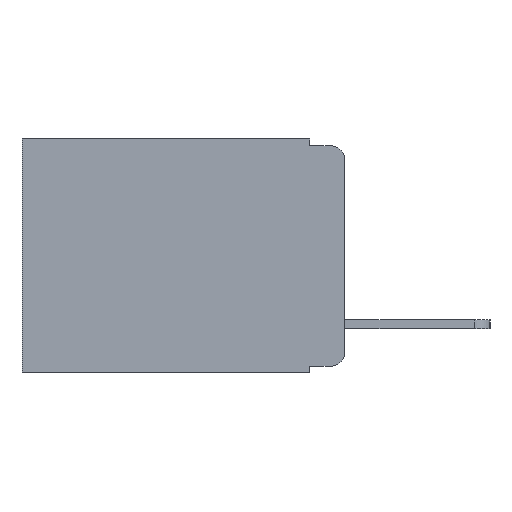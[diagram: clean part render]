
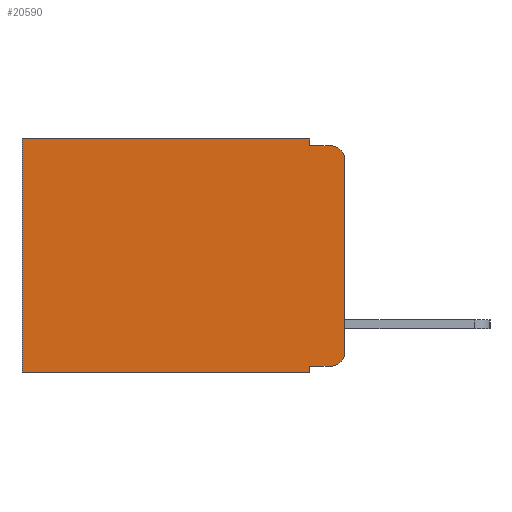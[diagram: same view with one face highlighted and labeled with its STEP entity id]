
A CAD part, left-side view. The second image highlights one B-rep face of the part: STEP entity #20590.
In plain terms, the highlighted planar face has unit normal (-1, 0, 0).
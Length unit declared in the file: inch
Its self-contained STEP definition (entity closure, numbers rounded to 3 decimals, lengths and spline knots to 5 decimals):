
#118 = CARTESIAN_POINT ( 'NONE',  ( 0.298, 0.051, -0.343 ) ) ;
#683 = CARTESIAN_POINT ( 'NONE',  ( 0.298, 0., 0. ) ) ;
#1264 = CARTESIAN_POINT ( 'NONE',  ( 0.298, 0.02, -0.03 ) ) ;
#1392 = VERTEX_POINT ( 'NONE', #2136 ) ;
#1413 = CARTESIAN_POINT ( 'NONE',  ( 0.298, 0.051, 0. ) ) ;
#1596 = CARTESIAN_POINT ( 'NONE',  ( 0.298, 0.051, -0.333 ) ) ;
#1978 = VERTEX_POINT ( 'NONE', #17481 ) ;
#2136 = CARTESIAN_POINT ( 'NONE',  ( 0.298, 0., -0.03 ) ) ;
#2285 = VERTEX_POINT ( 'NONE', #7405 ) ;
#2499 = VERTEX_POINT ( 'NONE', #1596 ) ;
#2525 = VERTEX_POINT ( 'NONE', #118 ) ;
#2598 = DIRECTION ( 'NONE',  ( 1., 0., 0. ) ) ;
#2883 = VERTEX_POINT ( 'NONE', #4368 ) ;
#3178 = DIRECTION ( 'NONE',  ( 0., 0., -1. ) ) ;
#3621 = EDGE_CURVE ( 'NONE', #1392, #4346, #22927, .T. ) ;
#4268 = EDGE_CURVE ( 'NONE', #1978, #2285, #23722, .T. ) ;
#4346 = VERTEX_POINT ( 'NONE', #17347 ) ;
#4368 = CARTESIAN_POINT ( 'NONE',  ( 0.298, 0.02, -0.01 ) ) ;
#4862 = AXIS2_PLACEMENT_3D ( 'NONE', #1264, #14166, #3178 ) ;
#5777 = DIRECTION ( 'NONE',  ( -1., 0., 0. ) ) ;
#5985 = VERTEX_POINT ( 'NONE', #17454 ) ;
#5993 = VECTOR ( 'NONE', #10094, 39.37008 ) ;
#6064 = CARTESIAN_POINT ( 'NONE',  ( 0.298, 0., 0. ) ) ;
#6790 = ORIENTED_EDGE ( 'NONE', *, *, #21470, .F. ) ;
#7341 = LINE ( 'NONE', #1413, #7925 ) ;
#7405 = CARTESIAN_POINT ( 'NONE',  ( 0.298, 0.051, -0.01 ) ) ;
#7545 = DIRECTION ( 'NONE',  ( 0., -1., 0. ) ) ;
#7668 = ORIENTED_EDGE ( 'NONE', *, *, #10254, .T. ) ;
#7925 = VECTOR ( 'NONE', #12558, 39.37008 ) ;
#7977 = VECTOR ( 'NONE', #22527, 39.37008 ) ;
#8647 = VECTOR ( 'NONE', #11410, 39.37008 ) ;
#8890 = VERTEX_POINT ( 'NONE', #18464 ) ;
#9008 = CIRCLE ( 'NONE', #21976, 0.02 ) ;
#9126 = ORIENTED_EDGE ( 'NONE', *, *, #12071, .F. ) ;
#9365 = VECTOR ( 'NONE', #10561, 39.37008 ) ;
#9601 = LINE ( 'NONE', #20122, #23371 ) ;
#10094 = DIRECTION ( 'NONE',  ( 0., 1., 0. ) ) ;
#10226 = ORIENTED_EDGE ( 'NONE', *, *, #3621, .F. ) ;
#10254 = EDGE_CURVE ( 'NONE', #1978, #8890, #20470, .T. ) ;
#10561 = DIRECTION ( 'NONE',  ( 0., 0., -1. ) ) ;
#11187 = DIRECTION ( 'NONE',  ( 0., 0., -1. ) ) ;
#11410 = DIRECTION ( 'NONE',  ( 0., -1., 0. ) ) ;
#12071 = EDGE_CURVE ( 'NONE', #2499, #2525, #7341, .T. ) ;
#12368 = VECTOR ( 'NONE', #7545, 39.37008 ) ;
#12472 = VECTOR ( 'NONE', #17918, 39.37008 ) ;
#12558 = DIRECTION ( 'NONE',  ( 0., 0., -1. ) ) ;
#13449 = LINE ( 'NONE', #16721, #8647 ) ;
#13624 = PLANE ( 'NONE',  #21069 ) ;
#13913 = EDGE_CURVE ( 'NONE', #2285, #2883, #22496, .T. ) ;
#13936 = CIRCLE ( 'NONE', #4862, 0.02 ) ;
#14166 = DIRECTION ( 'NONE',  ( -1., 0., 0. ) ) ;
#14914 = FACE_OUTER_BOUND ( 'NONE', #20981, .T. ) ;
#15218 = CARTESIAN_POINT ( 'NONE',  ( 0.298, 0.051, 0. ) ) ;
#15366 = DIRECTION ( 'NONE',  ( 0., 0., -1. ) ) ;
#16037 = CARTESIAN_POINT ( 'NONE',  ( 0.298, 0., -0.343 ) ) ;
#16562 = CARTESIAN_POINT ( 'NONE',  ( 0.298, 0.02, -0.313 ) ) ;
#16616 = EDGE_CURVE ( 'NONE', #2499, #18191, #13449, .T. ) ;
#16667 = ORIENTED_EDGE ( 'NONE', *, *, #17496, .T. ) ;
#16721 = CARTESIAN_POINT ( 'NONE',  ( 0.298, 0.051, -0.333 ) ) ;
#17155 = LINE ( 'NONE', #16037, #12472 ) ;
#17347 = CARTESIAN_POINT ( 'NONE',  ( 0.298, 0., -0.313 ) ) ;
#17454 = CARTESIAN_POINT ( 'NONE',  ( 0.298, 0.473, -0.343 ) ) ;
#17481 = CARTESIAN_POINT ( 'NONE',  ( 0.298, 0.051, 0. ) ) ;
#17496 = EDGE_CURVE ( 'NONE', #1392, #2883, #13936, .T. ) ;
#17518 = ORIENTED_EDGE ( 'NONE', *, *, #22434, .T. ) ;
#17918 = DIRECTION ( 'NONE',  ( 0., 1., 0. ) ) ;
#18191 = VERTEX_POINT ( 'NONE', #19770 ) ;
#18449 = DIRECTION ( 'NONE',  ( 0., 0., -1. ) ) ;
#18464 = CARTESIAN_POINT ( 'NONE',  ( 0.298, 0.473, 0. ) ) ;
#19770 = CARTESIAN_POINT ( 'NONE',  ( 0.298, 0.02, -0.333 ) ) ;
#20122 = CARTESIAN_POINT ( 'NONE',  ( 0.298, 0.473, 0. ) ) ;
#20470 = LINE ( 'NONE', #6064, #5993 ) ;
#20590 = ADVANCED_FACE ( 'NONE', ( #14914 ), #13624, .F. ) ;
#20977 = ORIENTED_EDGE ( 'NONE', *, *, #16616, .T. ) ;
#20981 = EDGE_LOOP ( 'NONE', ( #10226, #16667, #23161, #22897, #7668, #17518, #6790, #9126, #20977, #22345 ) ) ;
#21069 = AXIS2_PLACEMENT_3D ( 'NONE', #683, #2598, #15366 ) ;
#21455 = CARTESIAN_POINT ( 'NONE',  ( 0.298, 0., 0. ) ) ;
#21470 = EDGE_CURVE ( 'NONE', #2525, #5985, #17155, .T. ) ;
#21976 = AXIS2_PLACEMENT_3D ( 'NONE', #16562, #5777, #18449 ) ;
#22345 = ORIENTED_EDGE ( 'NONE', *, *, #22465, .T. ) ;
#22434 = EDGE_CURVE ( 'NONE', #8890, #5985, #9601, .T. ) ;
#22465 = EDGE_CURVE ( 'NONE', #18191, #4346, #9008, .T. ) ;
#22496 = LINE ( 'NONE', #23698, #12368 ) ;
#22527 = DIRECTION ( 'NONE',  ( 0., 0., -1. ) ) ;
#22897 = ORIENTED_EDGE ( 'NONE', *, *, #4268, .F. ) ;
#22927 = LINE ( 'NONE', #21455, #7977 ) ;
#23161 = ORIENTED_EDGE ( 'NONE', *, *, #13913, .F. ) ;
#23371 = VECTOR ( 'NONE', #11187, 39.37008 ) ;
#23698 = CARTESIAN_POINT ( 'NONE',  ( 0.298, 0.051, -0.01 ) ) ;
#23722 = LINE ( 'NONE', #15218, #9365 ) ;
